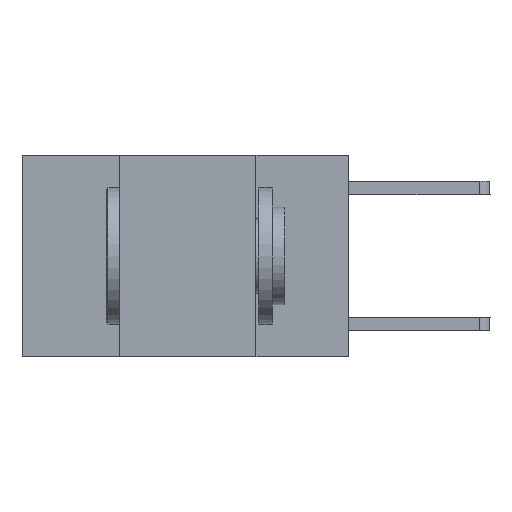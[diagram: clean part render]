
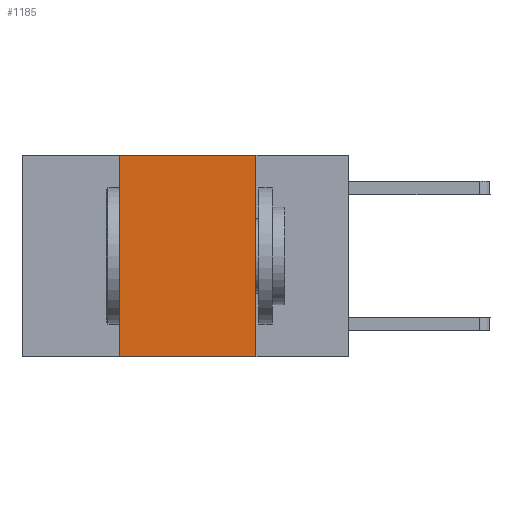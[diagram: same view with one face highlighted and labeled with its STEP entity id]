
A CAD part, left-side view. The second image highlights one B-rep face of the part: STEP entity #1185.
In plain terms, the highlighted planar face has unit normal (-1, 0, 0).
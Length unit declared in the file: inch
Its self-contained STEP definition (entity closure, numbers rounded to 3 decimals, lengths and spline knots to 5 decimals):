
#325 = EDGE_CURVE ( 'NONE', #10422, #522, #9790, .T. ) ;
#522 = VERTEX_POINT ( 'NONE', #3558 ) ;
#695 = LINE ( 'NONE', #9488, #10707 ) ;
#1167 = CARTESIAN_POINT ( 'NONE',  ( 0., 0.17, 0. ) ) ;
#1185 = ADVANCED_FACE ( 'NONE', ( #2246 ), #9974, .F. ) ;
#1281 = CARTESIAN_POINT ( 'NONE',  ( 0., 0.6, 0. ) ) ;
#1569 = CARTESIAN_POINT ( 'NONE',  ( 0., 0.6, 0. ) ) ;
#2083 = EDGE_LOOP ( 'NONE', ( #8803, #7184, #10397, #11226 ) ) ;
#2246 = FACE_OUTER_BOUND ( 'NONE', #2083, .T. ) ;
#2356 = VECTOR ( 'NONE', #5532, 39.37008 ) ;
#3558 = CARTESIAN_POINT ( 'NONE',  ( 0., 0.17, -0.37 ) ) ;
#3714 = EDGE_CURVE ( 'NONE', #7585, #10422, #7320, .T. ) ;
#3799 = CARTESIAN_POINT ( 'NONE',  ( 0., 0.42, 0. ) ) ;
#3827 = DIRECTION ( 'NONE',  ( 0., 0., -1. ) ) ;
#4308 = DIRECTION ( 'NONE',  ( 0., 0., -1. ) ) ;
#5532 = DIRECTION ( 'NONE',  ( 0., -1., 0. ) ) ;
#6565 = EDGE_CURVE ( 'NONE', #8721, #522, #695, .T. ) ;
#6958 = VECTOR ( 'NONE', #11352, 39.37008 ) ;
#7184 = ORIENTED_EDGE ( 'NONE', *, *, #3714, .F. ) ;
#7320 = LINE ( 'NONE', #1569, #2356 ) ;
#7329 = AXIS2_PLACEMENT_3D ( 'NONE', #1281, #8056, #4308 ) ;
#7585 = VERTEX_POINT ( 'NONE', #3799 ) ;
#8056 = DIRECTION ( 'NONE',  ( 1., 0., 0. ) ) ;
#8634 = CARTESIAN_POINT ( 'NONE',  ( 0., 0.42, 0. ) ) ;
#8721 = VERTEX_POINT ( 'NONE', #9337 ) ;
#8803 = ORIENTED_EDGE ( 'NONE', *, *, #325, .F. ) ;
#8827 = CARTESIAN_POINT ( 'NONE',  ( 0., 0.17, 0. ) ) ;
#9337 = CARTESIAN_POINT ( 'NONE',  ( 0., 0.42, -0.37 ) ) ;
#9338 = EDGE_CURVE ( 'NONE', #8721, #7585, #10537, .T. ) ;
#9488 = CARTESIAN_POINT ( 'NONE',  ( 0., 0.6, -0.37 ) ) ;
#9552 = DIRECTION ( 'NONE',  ( 0., -1., 0. ) ) ;
#9680 = VECTOR ( 'NONE', #3827, 39.37008 ) ;
#9790 = LINE ( 'NONE', #1167, #9680 ) ;
#9974 = PLANE ( 'NONE',  #7329 ) ;
#10397 = ORIENTED_EDGE ( 'NONE', *, *, #9338, .F. ) ;
#10422 = VERTEX_POINT ( 'NONE', #8827 ) ;
#10537 = LINE ( 'NONE', #8634, #6958 ) ;
#10707 = VECTOR ( 'NONE', #9552, 39.37008 ) ;
#11226 = ORIENTED_EDGE ( 'NONE', *, *, #6565, .T. ) ;
#11352 = DIRECTION ( 'NONE',  ( 0., 0., 1. ) ) ;
